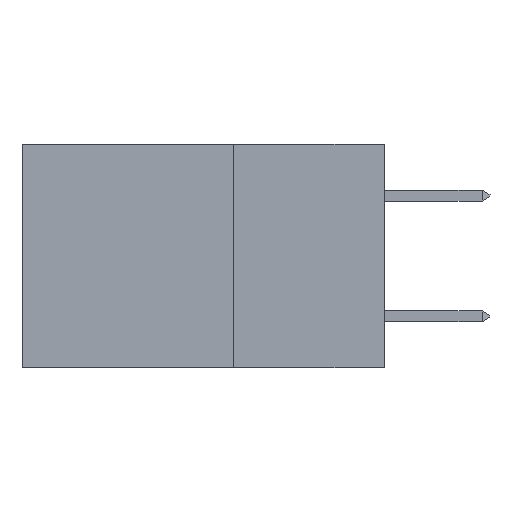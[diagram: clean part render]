
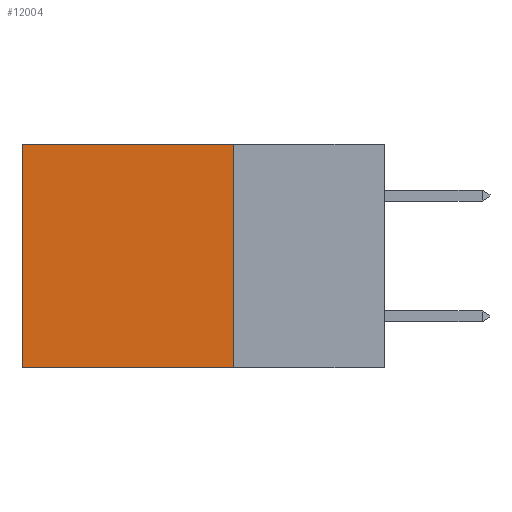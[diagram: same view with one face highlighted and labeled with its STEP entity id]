
A CAD part, left-side view. The second image highlights one B-rep face of the part: STEP entity #12004.
In plain terms, the highlighted planar face has unit normal (-1, 0, 0).
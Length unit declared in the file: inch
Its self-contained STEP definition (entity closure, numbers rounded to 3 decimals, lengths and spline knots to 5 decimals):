
#452 = CARTESIAN_POINT ( 'NONE',  ( 0.2875, 0.25, 0. ) ) ;
#578 = ORIENTED_EDGE ( 'NONE', *, *, #1684, .T. ) ;
#822 = DIRECTION ( 'NONE',  ( 0., 1., 0. ) ) ;
#1168 = ORIENTED_EDGE ( 'NONE', *, *, #11730, .T. ) ;
#1321 = ORIENTED_EDGE ( 'NONE', *, *, #22443, .F. ) ;
#1363 = DIRECTION ( 'NONE',  ( 0., 0., -1. ) ) ;
#1617 = EDGE_CURVE ( 'NONE', #5697, #18704, #18918, .T. ) ;
#1684 = EDGE_CURVE ( 'NONE', #5697, #14211, #12485, .T. ) ;
#3524 = VECTOR ( 'NONE', #4785, 39.37008 ) ;
#4785 = DIRECTION ( 'NONE',  ( 0., 1., 0. ) ) ;
#4992 = DIRECTION ( 'NONE',  ( 0., 0., -1. ) ) ;
#5697 = VERTEX_POINT ( 'NONE', #15309 ) ;
#6453 = VECTOR ( 'NONE', #1363, 39.37008 ) ;
#6497 = CARTESIAN_POINT ( 'NONE',  ( 0.2875, 0.25, 0. ) ) ;
#7296 = CARTESIAN_POINT ( 'NONE',  ( 0.2875, 0.6, -0.37 ) ) ;
#8716 = FACE_OUTER_BOUND ( 'NONE', #18676, .T. ) ;
#9833 = DIRECTION ( 'NONE',  ( 0., 0., -1. ) ) ;
#11458 = VERTEX_POINT ( 'NONE', #7296 ) ;
#11730 = EDGE_CURVE ( 'NONE', #14211, #11458, #23384, .T. ) ;
#12004 = ADVANCED_FACE ( 'NONE', ( #8716 ), #23668, .F. ) ;
#12485 = LINE ( 'NONE', #6497, #22912 ) ;
#14211 = VERTEX_POINT ( 'NONE', #22426 ) ;
#15309 = CARTESIAN_POINT ( 'NONE',  ( 0.2875, 0.25, 0. ) ) ;
#17199 = CARTESIAN_POINT ( 'NONE',  ( 0.2875, 0.25, -0.37 ) ) ;
#17760 = DIRECTION ( 'NONE',  ( 1., 0., 0. ) ) ;
#18172 = VECTOR ( 'NONE', #4992, 39.37008 ) ;
#18676 = EDGE_LOOP ( 'NONE', ( #1168, #1321, #23571, #578 ) ) ;
#18704 = VERTEX_POINT ( 'NONE', #17199 ) ;
#18711 = CARTESIAN_POINT ( 'NONE',  ( 0.2875, 0.6, 0. ) ) ;
#18848 = CARTESIAN_POINT ( 'NONE',  ( 0.2875, 0.25, -0.37 ) ) ;
#18918 = LINE ( 'NONE', #452, #6453 ) ;
#19706 = LINE ( 'NONE', #18848, #3524 ) ;
#21451 = CARTESIAN_POINT ( 'NONE',  ( 0.2875, 0.25, 0. ) ) ;
#22426 = CARTESIAN_POINT ( 'NONE',  ( 0.2875, 0.6, 0. ) ) ;
#22443 = EDGE_CURVE ( 'NONE', #18704, #11458, #19706, .T. ) ;
#22722 = AXIS2_PLACEMENT_3D ( 'NONE', #21451, #17760, #9833 ) ;
#22912 = VECTOR ( 'NONE', #822, 39.37008 ) ;
#23384 = LINE ( 'NONE', #18711, #18172 ) ;
#23571 = ORIENTED_EDGE ( 'NONE', *, *, #1617, .F. ) ;
#23668 = PLANE ( 'NONE',  #22722 ) ;
